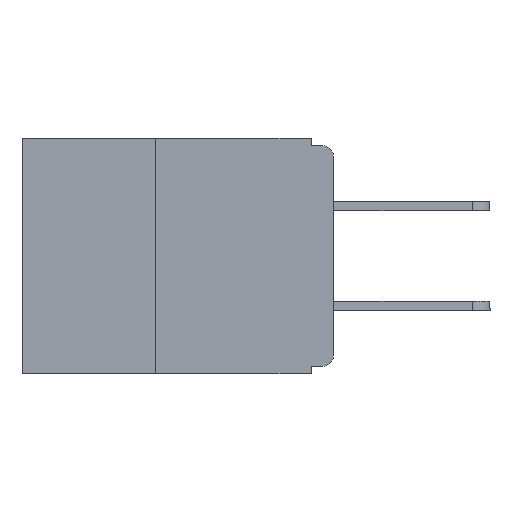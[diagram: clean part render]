
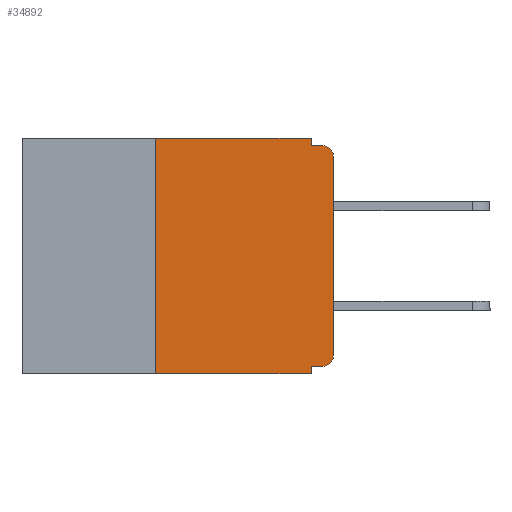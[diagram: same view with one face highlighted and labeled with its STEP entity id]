
A CAD part, left-side view. The second image highlights one B-rep face of the part: STEP entity #34892.
In plain terms, the highlighted planar face has unit normal (-1, 0, 0).
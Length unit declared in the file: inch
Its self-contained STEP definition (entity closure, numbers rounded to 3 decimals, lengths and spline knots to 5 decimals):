
#93 = PLANE ( 'NONE',  #6904 ) ;
#281 = CARTESIAN_POINT ( 'NONE',  ( 0., 0.25, -0.33 ) ) ;
#959 = CARTESIAN_POINT ( 'NONE',  ( 0., 0., 0. ) ) ;
#1145 = CARTESIAN_POINT ( 'NONE',  ( 0., 0.437, -0.33 ) ) ;
#1785 = DIRECTION ( 'NONE',  ( 0., -1., 0. ) ) ;
#1916 = CARTESIAN_POINT ( 'NONE',  ( 0., 0.031, 0. ) ) ;
#2906 = ORIENTED_EDGE ( 'NONE', *, *, #4833, .T. ) ;
#2976 = CARTESIAN_POINT ( 'NONE',  ( 0., 0., -0.01 ) ) ;
#4248 = CARTESIAN_POINT ( 'NONE',  ( 0., 0.015, -0.305 ) ) ;
#4545 = CARTESIAN_POINT ( 'NONE',  ( 0., 0.015, -0.025 ) ) ;
#4711 = EDGE_CURVE ( 'NONE', #7789, #23809, #7343, .T. ) ;
#4833 = EDGE_CURVE ( 'NONE', #33809, #11544, #16962, .T. ) ;
#5685 = LINE ( 'NONE', #30075, #26990 ) ;
#6026 = VECTOR ( 'NONE', #26546, 39.37008 ) ;
#6439 = VECTOR ( 'NONE', #1785, 39.37008 ) ;
#6441 = LINE ( 'NONE', #23351, #34037 ) ;
#6710 = VERTEX_POINT ( 'NONE', #32297 ) ;
#6774 = VERTEX_POINT ( 'NONE', #29689 ) ;
#6904 = AXIS2_PLACEMENT_3D ( 'NONE', #14206, #25182, #19868 ) ;
#7138 = DIRECTION ( 'NONE',  ( 0., 0., -1. ) ) ;
#7343 = LINE ( 'NONE', #1145, #6439 ) ;
#7435 = DIRECTION ( 'NONE',  ( 0., 0., -1. ) ) ;
#7575 = FACE_OUTER_BOUND ( 'NONE', #27035, .T. ) ;
#7789 = VERTEX_POINT ( 'NONE', #26024 ) ;
#8118 = ORIENTED_EDGE ( 'NONE', *, *, #24050, .F. ) ;
#8203 = ORIENTED_EDGE ( 'NONE', *, *, #17758, .F. ) ;
#8669 = ORIENTED_EDGE ( 'NONE', *, *, #4711, .T. ) ;
#8882 = VECTOR ( 'NONE', #22752, 39.37008 ) ;
#9528 = VECTOR ( 'NONE', #35650, 39.37008 ) ;
#9850 = VERTEX_POINT ( 'NONE', #16105 ) ;
#9975 = CARTESIAN_POINT ( 'NONE',  ( 0., 0., -0.32 ) ) ;
#11400 = ORIENTED_EDGE ( 'NONE', *, *, #15435, .F. ) ;
#11503 = CARTESIAN_POINT ( 'NONE',  ( 0., 0.031, -0.33 ) ) ;
#11544 = VERTEX_POINT ( 'NONE', #34940 ) ;
#11620 = CARTESIAN_POINT ( 'NONE',  ( 0., 0.437, 0. ) ) ;
#12324 = EDGE_CURVE ( 'NONE', #11544, #14894, #25488, .T. ) ;
#12362 = VERTEX_POINT ( 'NONE', #1916 ) ;
#13074 = AXIS2_PLACEMENT_3D ( 'NONE', #4248, #23778, #7138 ) ;
#14049 = EDGE_CURVE ( 'NONE', #12362, #6710, #6441, .T. ) ;
#14206 = CARTESIAN_POINT ( 'NONE',  ( 0., 0.437, 0. ) ) ;
#14894 = VERTEX_POINT ( 'NONE', #16219 ) ;
#15127 = DIRECTION ( 'NONE',  ( 0., 0., -1. ) ) ;
#15394 = EDGE_CURVE ( 'NONE', #6710, #14894, #20363, .T. ) ;
#15435 = EDGE_CURVE ( 'NONE', #6774, #12362, #18647, .T. ) ;
#15966 = ORIENTED_EDGE ( 'NONE', *, *, #14049, .F. ) ;
#16105 = CARTESIAN_POINT ( 'NONE',  ( 0., 0.031, -0.32 ) ) ;
#16219 = CARTESIAN_POINT ( 'NONE',  ( 0., 0.015, -0.01 ) ) ;
#16962 = LINE ( 'NONE', #959, #9528 ) ;
#17030 = DIRECTION ( 'NONE',  ( 0., -1., 0. ) ) ;
#17758 = EDGE_CURVE ( 'NONE', #9850, #23809, #5685, .T. ) ;
#18647 = LINE ( 'NONE', #11620, #34783 ) ;
#19015 = ORIENTED_EDGE ( 'NONE', *, *, #15394, .F. ) ;
#19416 = AXIS2_PLACEMENT_3D ( 'NONE', #4545, #24067, #7435 ) ;
#19868 = DIRECTION ( 'NONE',  ( 0., 0., -1. ) ) ;
#20214 = EDGE_CURVE ( 'NONE', #26611, #9850, #21796, .T. ) ;
#20363 = LINE ( 'NONE', #2976, #26758 ) ;
#21796 = LINE ( 'NONE', #9975, #6026 ) ;
#22524 = ORIENTED_EDGE ( 'NONE', *, *, #12324, .T. ) ;
#22752 = DIRECTION ( 'NONE',  ( 0., 0., 1. ) ) ;
#23351 = CARTESIAN_POINT ( 'NONE',  ( 0., 0.031, 0. ) ) ;
#23778 = DIRECTION ( 'NONE',  ( -1., 0., 0. ) ) ;
#23809 = VERTEX_POINT ( 'NONE', #11503 ) ;
#24050 = EDGE_CURVE ( 'NONE', #7789, #6774, #30910, .T. ) ;
#24067 = DIRECTION ( 'NONE',  ( -1., 0., 0. ) ) ;
#25182 = DIRECTION ( 'NONE',  ( 1., 0., 0. ) ) ;
#25488 = CIRCLE ( 'NONE', #19416, 0.015 ) ;
#26024 = CARTESIAN_POINT ( 'NONE',  ( 0., 0.25, -0.33 ) ) ;
#26546 = DIRECTION ( 'NONE',  ( 0., 1., 0. ) ) ;
#26611 = VERTEX_POINT ( 'NONE', #30695 ) ;
#26758 = VECTOR ( 'NONE', #17030, 39.37008 ) ;
#26990 = VECTOR ( 'NONE', #32795, 39.37008 ) ;
#27035 = EDGE_LOOP ( 'NONE', ( #2906, #22524, #19015, #15966, #11400, #8118, #8669, #8203, #30787, #32214 ) ) ;
#29689 = CARTESIAN_POINT ( 'NONE',  ( 0., 0.25, 0. ) ) ;
#30075 = CARTESIAN_POINT ( 'NONE',  ( 0., 0.031, -0.33 ) ) ;
#30695 = CARTESIAN_POINT ( 'NONE',  ( 0., 0.015, -0.32 ) ) ;
#30787 = ORIENTED_EDGE ( 'NONE', *, *, #20214, .F. ) ;
#30910 = LINE ( 'NONE', #281, #8882 ) ;
#30919 = DIRECTION ( 'NONE',  ( 0., -1., 0. ) ) ;
#31559 = CIRCLE ( 'NONE', #13074, 0.015 ) ;
#32214 = ORIENTED_EDGE ( 'NONE', *, *, #32726, .T. ) ;
#32297 = CARTESIAN_POINT ( 'NONE',  ( 0., 0.031, -0.01 ) ) ;
#32726 = EDGE_CURVE ( 'NONE', #26611, #33809, #31559, .T. ) ;
#32795 = DIRECTION ( 'NONE',  ( 0., 0., -1. ) ) ;
#33809 = VERTEX_POINT ( 'NONE', #34260 ) ;
#34037 = VECTOR ( 'NONE', #15127, 39.37008 ) ;
#34260 = CARTESIAN_POINT ( 'NONE',  ( 0., 0., -0.305 ) ) ;
#34783 = VECTOR ( 'NONE', #30919, 39.37008 ) ;
#34892 = ADVANCED_FACE ( 'NONE', ( #7575 ), #93, .F. ) ;
#34940 = CARTESIAN_POINT ( 'NONE',  ( 0., 0., -0.025 ) ) ;
#35650 = DIRECTION ( 'NONE',  ( 0., 0., 1. ) ) ;
